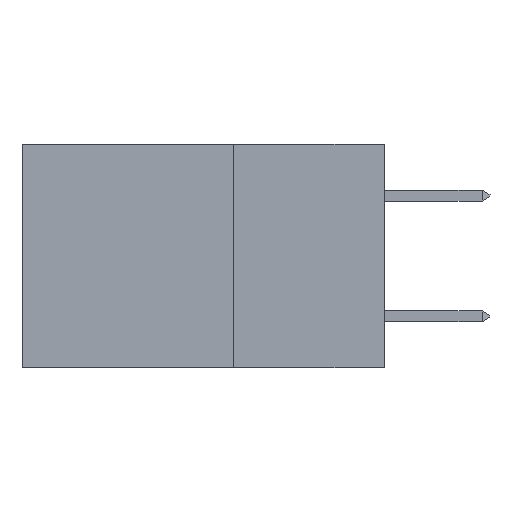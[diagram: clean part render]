
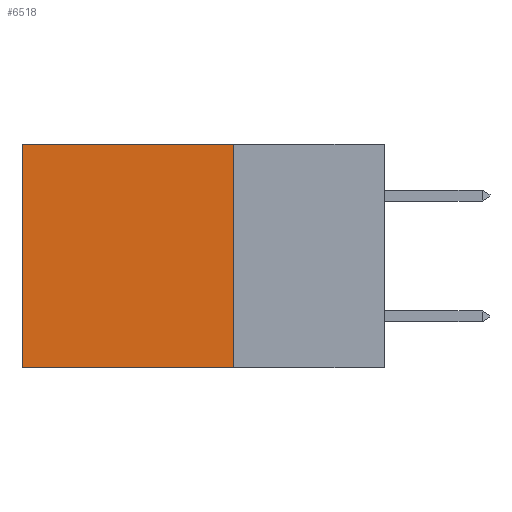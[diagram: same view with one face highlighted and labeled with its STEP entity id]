
A CAD part, left-side view. The second image highlights one B-rep face of the part: STEP entity #6518.
In plain terms, the highlighted planar face has unit normal (-1, 0, 0).
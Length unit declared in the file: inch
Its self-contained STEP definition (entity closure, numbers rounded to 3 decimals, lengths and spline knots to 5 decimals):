
#216 = PLANE ( 'NONE',  #11767 ) ;
#903 = ORIENTED_EDGE ( 'NONE', *, *, #2074, .F. ) ;
#1656 = CARTESIAN_POINT ( 'NONE',  ( 0.2875, 0.25, -0.37 ) ) ;
#1830 = CARTESIAN_POINT ( 'NONE',  ( 0.2875, 0.6, 0. ) ) ;
#2074 = EDGE_CURVE ( 'NONE', #2257, #3825, #10992, .T. ) ;
#2257 = VERTEX_POINT ( 'NONE', #7416 ) ;
#2475 = CARTESIAN_POINT ( 'NONE',  ( 0.2875, 0.6, 0. ) ) ;
#2619 = EDGE_CURVE ( 'NONE', #12435, #10130, #13103, .T. ) ;
#2875 = DIRECTION ( 'NONE',  ( 0., 1., 0. ) ) ;
#2978 = DIRECTION ( 'NONE',  ( 0., 0., -1. ) ) ;
#3164 = DIRECTION ( 'NONE',  ( 0., 0., -1. ) ) ;
#3634 = VECTOR ( 'NONE', #13448, 39.37008 ) ;
#3825 = VERTEX_POINT ( 'NONE', #1656 ) ;
#5902 = LINE ( 'NONE', #13990, #16067 ) ;
#6307 = DIRECTION ( 'NONE',  ( 0., 1., 0. ) ) ;
#6518 = ADVANCED_FACE ( 'NONE', ( #14540 ), #216, .F. ) ;
#7416 = CARTESIAN_POINT ( 'NONE',  ( 0.2875, 0.25, 0. ) ) ;
#7930 = ORIENTED_EDGE ( 'NONE', *, *, #13177, .F. ) ;
#8392 = CARTESIAN_POINT ( 'NONE',  ( 0.2875, 0.25, 0. ) ) ;
#9347 = CARTESIAN_POINT ( 'NONE',  ( 0.2875, 0.25, 0. ) ) ;
#9459 = CARTESIAN_POINT ( 'NONE',  ( 0.2875, 0.25, 0. ) ) ;
#9681 = EDGE_LOOP ( 'NONE', ( #12067, #7930, #903, #15851 ) ) ;
#10130 = VERTEX_POINT ( 'NONE', #14769 ) ;
#10782 = DIRECTION ( 'NONE',  ( 1., 0., 0. ) ) ;
#10992 = LINE ( 'NONE', #8392, #14302 ) ;
#11310 = VECTOR ( 'NONE', #2875, 39.37008 ) ;
#11767 = AXIS2_PLACEMENT_3D ( 'NONE', #9459, #10782, #2978 ) ;
#12067 = ORIENTED_EDGE ( 'NONE', *, *, #2619, .T. ) ;
#12435 = VERTEX_POINT ( 'NONE', #2475 ) ;
#13103 = LINE ( 'NONE', #1830, #3634 ) ;
#13177 = EDGE_CURVE ( 'NONE', #3825, #10130, #5902, .T. ) ;
#13448 = DIRECTION ( 'NONE',  ( 0., 0., -1. ) ) ;
#13990 = CARTESIAN_POINT ( 'NONE',  ( 0.2875, 0.25, -0.37 ) ) ;
#14302 = VECTOR ( 'NONE', #3164, 39.37008 ) ;
#14540 = FACE_OUTER_BOUND ( 'NONE', #9681, .T. ) ;
#14769 = CARTESIAN_POINT ( 'NONE',  ( 0.2875, 0.6, -0.37 ) ) ;
#15401 = LINE ( 'NONE', #9347, #11310 ) ;
#15851 = ORIENTED_EDGE ( 'NONE', *, *, #16514, .T. ) ;
#16067 = VECTOR ( 'NONE', #6307, 39.37008 ) ;
#16514 = EDGE_CURVE ( 'NONE', #2257, #12435, #15401, .T. ) ;
